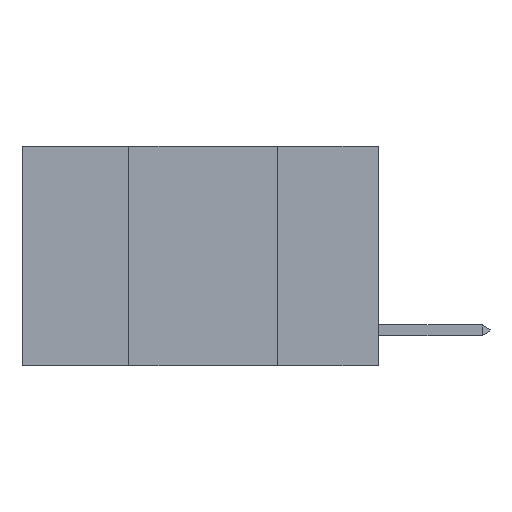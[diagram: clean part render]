
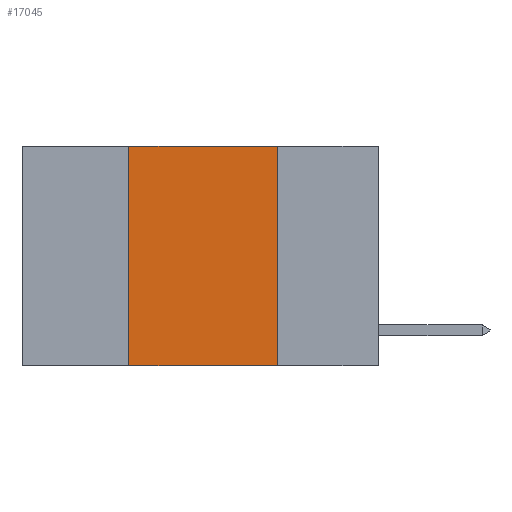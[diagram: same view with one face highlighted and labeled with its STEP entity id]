
A CAD part, left-side view. The second image highlights one B-rep face of the part: STEP entity #17045.
In plain terms, the highlighted planar face has unit normal (-1, 0, 0).
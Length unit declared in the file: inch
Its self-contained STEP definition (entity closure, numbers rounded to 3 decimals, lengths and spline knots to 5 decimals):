
#1379 = CARTESIAN_POINT ( 'NONE',  ( 0., 0.17, 0. ) ) ;
#2896 = VECTOR ( 'NONE', #8456, 39.37008 ) ;
#3338 = DIRECTION ( 'NONE',  ( 0., 0., -1. ) ) ;
#3565 = VERTEX_POINT ( 'NONE', #21454 ) ;
#3619 = ORIENTED_EDGE ( 'NONE', *, *, #5270, .F. ) ;
#4031 = LINE ( 'NONE', #12425, #14128 ) ;
#5270 = EDGE_CURVE ( 'NONE', #3565, #8463, #23550, .T. ) ;
#6342 = DIRECTION ( 'NONE',  ( 0., -1., 0. ) ) ;
#8119 = VERTEX_POINT ( 'NONE', #20501 ) ;
#8456 = DIRECTION ( 'NONE',  ( 0., -1., 0. ) ) ;
#8463 = VERTEX_POINT ( 'NONE', #23157 ) ;
#8644 = FACE_OUTER_BOUND ( 'NONE', #18908, .T. ) ;
#9292 = ORIENTED_EDGE ( 'NONE', *, *, #22541, .T. ) ;
#11004 = DIRECTION ( 'NONE',  ( 0., 0., -1. ) ) ;
#12425 = CARTESIAN_POINT ( 'NONE',  ( 0., 0.42, 0. ) ) ;
#12595 = VECTOR ( 'NONE', #3338, 39.37008 ) ;
#13622 = LINE ( 'NONE', #21922, #2896 ) ;
#14128 = VECTOR ( 'NONE', #16326, 39.37008 ) ;
#15683 = EDGE_CURVE ( 'NONE', #8463, #8119, #22873, .T. ) ;
#16326 = DIRECTION ( 'NONE',  ( 0., 0., 1. ) ) ;
#16717 = CARTESIAN_POINT ( 'NONE',  ( 0., 0.6, 0. ) ) ;
#17045 = ADVANCED_FACE ( 'NONE', ( #8644 ), #20624, .F. ) ;
#17101 = ORIENTED_EDGE ( 'NONE', *, *, #15683, .F. ) ;
#17840 = VECTOR ( 'NONE', #6342, 39.37008 ) ;
#18270 = AXIS2_PLACEMENT_3D ( 'NONE', #16717, #22520, #11004 ) ;
#18908 = EDGE_LOOP ( 'NONE', ( #17101, #3619, #18953, #9292 ) ) ;
#18953 = ORIENTED_EDGE ( 'NONE', *, *, #18982, .F. ) ;
#18982 = EDGE_CURVE ( 'NONE', #19891, #3565, #4031, .T. ) ;
#19891 = VERTEX_POINT ( 'NONE', #24564 ) ;
#20501 = CARTESIAN_POINT ( 'NONE',  ( 0., 0.17, -0.37 ) ) ;
#20624 = PLANE ( 'NONE',  #18270 ) ;
#21454 = CARTESIAN_POINT ( 'NONE',  ( 0., 0.42, 0. ) ) ;
#21922 = CARTESIAN_POINT ( 'NONE',  ( 0., 0.6, -0.37 ) ) ;
#22520 = DIRECTION ( 'NONE',  ( 1., 0., 0. ) ) ;
#22541 = EDGE_CURVE ( 'NONE', #19891, #8119, #13622, .T. ) ;
#22873 = LINE ( 'NONE', #1379, #12595 ) ;
#23157 = CARTESIAN_POINT ( 'NONE',  ( 0., 0.17, 0. ) ) ;
#23435 = CARTESIAN_POINT ( 'NONE',  ( 0., 0.6, 0. ) ) ;
#23550 = LINE ( 'NONE', #23435, #17840 ) ;
#24564 = CARTESIAN_POINT ( 'NONE',  ( 0., 0.42, -0.37 ) ) ;
